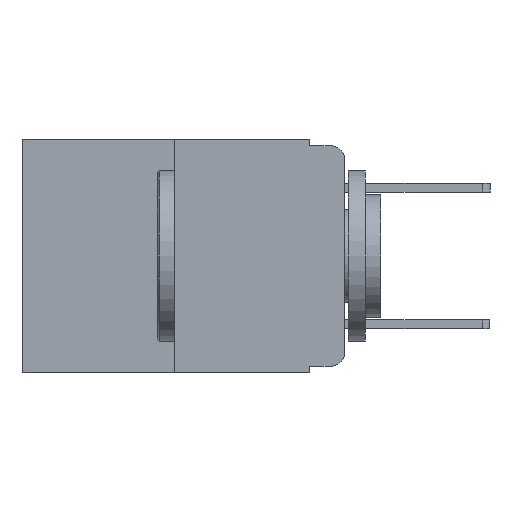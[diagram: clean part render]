
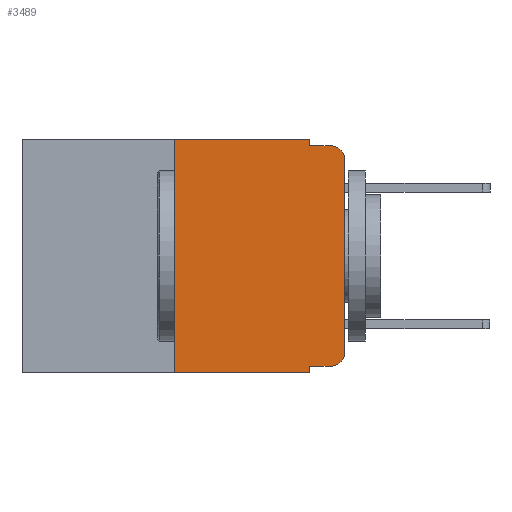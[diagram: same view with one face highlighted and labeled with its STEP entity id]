
A CAD part, left-side view. The second image highlights one B-rep face of the part: STEP entity #3489.
In plain terms, the highlighted planar face has unit normal (-1, 0, 0).
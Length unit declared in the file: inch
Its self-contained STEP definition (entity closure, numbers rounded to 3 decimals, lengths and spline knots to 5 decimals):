
#19 = CARTESIAN_POINT ( 'NONE',  ( 0., 0.02, -0.01 ) ) ;
#856 = VERTEX_POINT ( 'NONE', #19 ) ;
#1270 = VERTEX_POINT ( 'NONE', #11768 ) ;
#1418 = ORIENTED_EDGE ( 'NONE', *, *, #5626, .T. ) ;
#1534 = VECTOR ( 'NONE', #10392, 39.37008 ) ;
#1776 = VERTEX_POINT ( 'NONE', #4525 ) ;
#1814 = ORIENTED_EDGE ( 'NONE', *, *, #8248, .T. ) ;
#1832 = ORIENTED_EDGE ( 'NONE', *, *, #16207, .T. ) ;
#2002 = LINE ( 'NONE', #17042, #18797 ) ;
#2132 = VECTOR ( 'NONE', #18700, 39.37008 ) ;
#2388 = CARTESIAN_POINT ( 'NONE',  ( 0., 0.02, -0.03 ) ) ;
#2487 = DIRECTION ( 'NONE',  ( -1., 0., 0. ) ) ;
#2842 = VECTOR ( 'NONE', #16853, 39.37008 ) ;
#2933 = ORIENTED_EDGE ( 'NONE', *, *, #9312, .T. ) ;
#2987 = CARTESIAN_POINT ( 'NONE',  ( 0., 0.051, 0. ) ) ;
#3359 = FACE_OUTER_BOUND ( 'NONE', #11310, .T. ) ;
#3489 = ADVANCED_FACE ( 'NONE', ( #3359 ), #12433, .F. ) ;
#3626 = CARTESIAN_POINT ( 'NONE',  ( 0., 0.473, 0. ) ) ;
#3705 = DIRECTION ( 'NONE',  ( 0., -1., 0. ) ) ;
#3831 = CARTESIAN_POINT ( 'NONE',  ( 0., 0.25, -0.343 ) ) ;
#4197 = DIRECTION ( 'NONE',  ( 0., 0., -1. ) ) ;
#4379 = LINE ( 'NONE', #7892, #11851 ) ;
#4396 = CARTESIAN_POINT ( 'NONE',  ( 0., 0.051, -0.01 ) ) ;
#4525 = CARTESIAN_POINT ( 'NONE',  ( 0., 0.051, -0.01 ) ) ;
#4930 = CARTESIAN_POINT ( 'NONE',  ( 0., 0.25, 0. ) ) ;
#5219 = VECTOR ( 'NONE', #14187, 39.37008 ) ;
#5276 = CARTESIAN_POINT ( 'NONE',  ( 0., 0.051, 0. ) ) ;
#5461 = ORIENTED_EDGE ( 'NONE', *, *, #20354, .F. ) ;
#5626 = EDGE_CURVE ( 'NONE', #20273, #1270, #2002, .T. ) ;
#6157 = DIRECTION ( 'NONE',  ( 0., -1., 0. ) ) ;
#6240 = AXIS2_PLACEMENT_3D ( 'NONE', #12728, #2487, #14361 ) ;
#6242 = VERTEX_POINT ( 'NONE', #15819 ) ;
#6351 = ORIENTED_EDGE ( 'NONE', *, *, #18564, .F. ) ;
#6693 = CARTESIAN_POINT ( 'NONE',  ( 0., 0.02, -0.333 ) ) ;
#6858 = LINE ( 'NONE', #13804, #2132 ) ;
#7145 = DIRECTION ( 'NONE',  ( 0., 0., -1. ) ) ;
#7564 = LINE ( 'NONE', #5276, #2842 ) ;
#7787 = VECTOR ( 'NONE', #6157, 39.37008 ) ;
#7892 = CARTESIAN_POINT ( 'NONE',  ( 0., 0.051, 0. ) ) ;
#8248 = EDGE_CURVE ( 'NONE', #1270, #856, #16633, .T. ) ;
#8626 = EDGE_CURVE ( 'NONE', #6242, #14035, #6858, .T. ) ;
#9312 = EDGE_CURVE ( 'NONE', #14035, #20273, #17079, .T. ) ;
#9672 = DIRECTION ( 'NONE',  ( 0., 0., -1. ) ) ;
#9790 = EDGE_CURVE ( 'NONE', #14372, #10760, #18415, .T. ) ;
#10058 = VERTEX_POINT ( 'NONE', #2987 ) ;
#10341 = CARTESIAN_POINT ( 'NONE',  ( 0., 0.051, -0.343 ) ) ;
#10392 = DIRECTION ( 'NONE',  ( 0., -1., 0. ) ) ;
#10760 = VERTEX_POINT ( 'NONE', #4930 ) ;
#10972 = ORIENTED_EDGE ( 'NONE', *, *, #16562, .F. ) ;
#10992 = CARTESIAN_POINT ( 'NONE',  ( 0., 0.25, 0. ) ) ;
#11310 = EDGE_LOOP ( 'NONE', ( #1418, #1814, #5461, #6351, #15989, #19443, #1832, #10972, #12440, #2933 ) ) ;
#11768 = CARTESIAN_POINT ( 'NONE',  ( 0., 0., -0.03 ) ) ;
#11851 = VECTOR ( 'NONE', #9672, 39.37008 ) ;
#12433 = PLANE ( 'NONE',  #16871 ) ;
#12440 = ORIENTED_EDGE ( 'NONE', *, *, #8626, .T. ) ;
#12728 = CARTESIAN_POINT ( 'NONE',  ( 0., 0.02, -0.313 ) ) ;
#12756 = VECTOR ( 'NONE', #3705, 39.37008 ) ;
#13163 = EDGE_CURVE ( 'NONE', #10760, #10058, #18573, .T. ) ;
#13804 = CARTESIAN_POINT ( 'NONE',  ( 0., 0.051, -0.333 ) ) ;
#14035 = VERTEX_POINT ( 'NONE', #6693 ) ;
#14187 = DIRECTION ( 'NONE',  ( 0., 0., 1. ) ) ;
#14223 = CARTESIAN_POINT ( 'NONE',  ( 0., 0., -0.313 ) ) ;
#14262 = DIRECTION ( 'NONE',  ( -1., 0., 0. ) ) ;
#14361 = DIRECTION ( 'NONE',  ( 0., 0., -1. ) ) ;
#14372 = VERTEX_POINT ( 'NONE', #3831 ) ;
#15010 = DIRECTION ( 'NONE',  ( 1., 0., 0. ) ) ;
#15124 = LINE ( 'NONE', #20007, #1534 ) ;
#15609 = VERTEX_POINT ( 'NONE', #10341 ) ;
#15819 = CARTESIAN_POINT ( 'NONE',  ( 0., 0.051, -0.333 ) ) ;
#15989 = ORIENTED_EDGE ( 'NONE', *, *, #13163, .F. ) ;
#16207 = EDGE_CURVE ( 'NONE', #14372, #15609, #15124, .T. ) ;
#16562 = EDGE_CURVE ( 'NONE', #6242, #15609, #4379, .T. ) ;
#16633 = CIRCLE ( 'NONE', #17656, 0.02 ) ;
#16853 = DIRECTION ( 'NONE',  ( 0., 0., -1. ) ) ;
#16871 = AXIS2_PLACEMENT_3D ( 'NONE', #17034, #15010, #7145 ) ;
#17034 = CARTESIAN_POINT ( 'NONE',  ( 0., 0.473, 0. ) ) ;
#17042 = CARTESIAN_POINT ( 'NONE',  ( 0., 0., 0. ) ) ;
#17079 = CIRCLE ( 'NONE', #6240, 0.02 ) ;
#17656 = AXIS2_PLACEMENT_3D ( 'NONE', #2388, #14262, #4197 ) ;
#18415 = LINE ( 'NONE', #10992, #5219 ) ;
#18564 = EDGE_CURVE ( 'NONE', #10058, #1776, #7564, .T. ) ;
#18573 = LINE ( 'NONE', #3626, #12756 ) ;
#18700 = DIRECTION ( 'NONE',  ( 0., -1., 0. ) ) ;
#18797 = VECTOR ( 'NONE', #20908, 39.37008 ) ;
#19443 = ORIENTED_EDGE ( 'NONE', *, *, #9790, .F. ) ;
#20007 = CARTESIAN_POINT ( 'NONE',  ( 0., 0.473, -0.343 ) ) ;
#20273 = VERTEX_POINT ( 'NONE', #14223 ) ;
#20354 = EDGE_CURVE ( 'NONE', #1776, #856, #20776, .T. ) ;
#20776 = LINE ( 'NONE', #4396, #7787 ) ;
#20908 = DIRECTION ( 'NONE',  ( 0., 0., 1. ) ) ;
